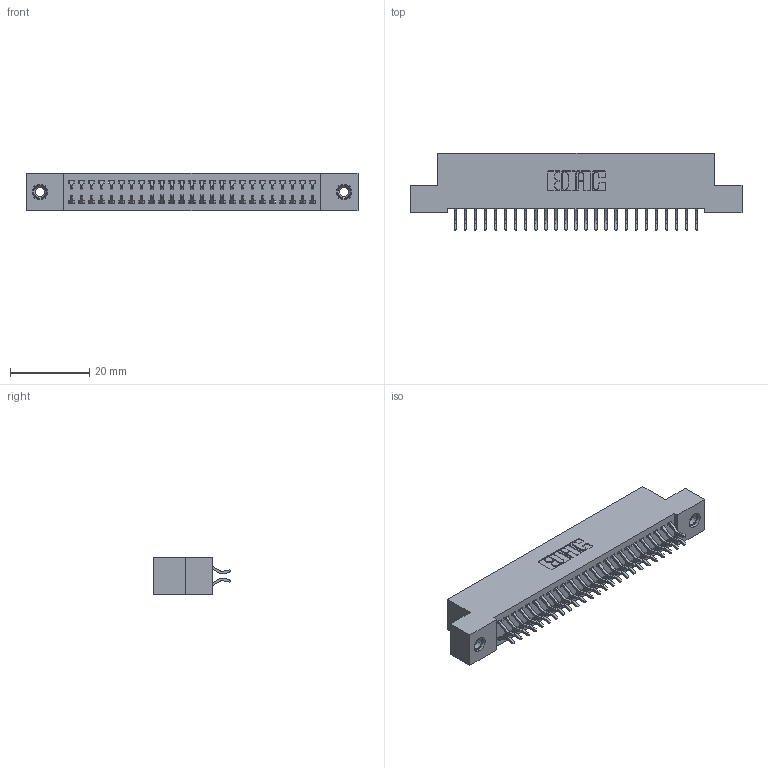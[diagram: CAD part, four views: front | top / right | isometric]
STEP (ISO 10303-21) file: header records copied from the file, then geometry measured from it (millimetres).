
FILE_DESCRIPTION (( 'STEP AP203' ), '1' );
FILE_NAME ('342-050-556-208.STEP', '2018-08-12T20:18:48', ( '' ), ( '' ), 'SwSTEP 2.0', 'SolidWorks 2016', '' );
FILE_SCHEMA (( 'CONFIG_CONTROL_DESIGN' ));
Length unit declared in the file: inch
Products named in the file (4): 345-250-001_345-250-003-102; 342-050-556-208; 342 Part_TI; 345-292-001_556 Tail
Assembly tree (53 placements, depth 2):
  342-050-556-208
    342 Part_TI
    345-292-001_556 Tail  x50
    345-250-001_345-250-003-102  x2
Bounding box: 83.82 x 19.58 x 9.4 mm (x, y, z)
Volume: 7443.8 mm3; surface area: 11659.5 mm2
Topology: 53 solids, 53 shells, 3070 faces, 9085 edges, 5982 vertices
Faces by surface type: plane 2098, cylinder 956, cone 12, torus 4
Entity records: 19556 total; most frequent: CARTESIAN_POINT 3257, ORIENTED_EDGE 3174, DIRECTION 2833, EDGE_CURVE 1587, VECTOR 1431, LINE 1431, VERTEX_POINT 1052, AXIS2_PLACEMENT_3D 701
